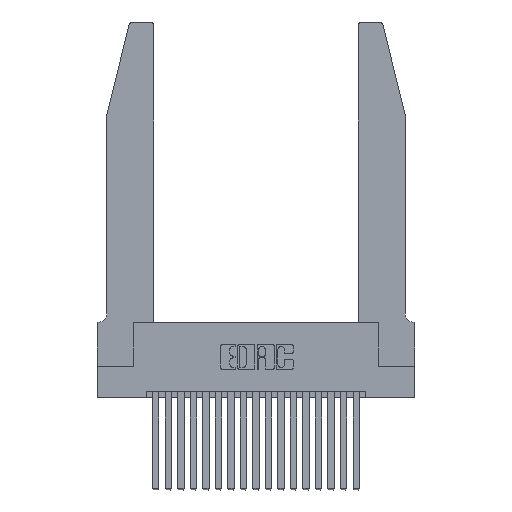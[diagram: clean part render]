
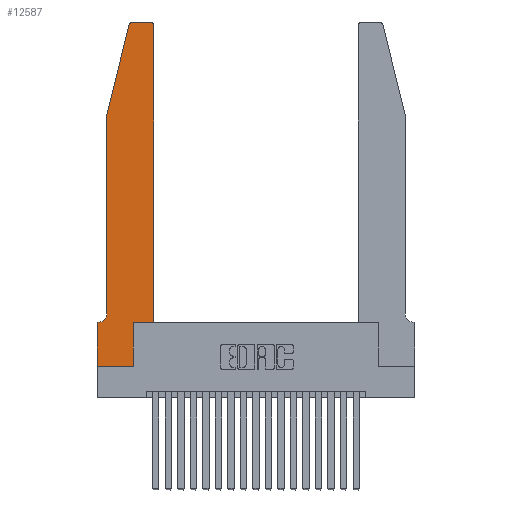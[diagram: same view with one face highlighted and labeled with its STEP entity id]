
A CAD part, top view. The second image highlights one B-rep face of the part: STEP entity #12587.
In plain terms, the highlighted planar face has unit normal (0, 0, 1).
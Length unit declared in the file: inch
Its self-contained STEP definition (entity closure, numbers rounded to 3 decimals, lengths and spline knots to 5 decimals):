
#90 = AXIS2_PLACEMENT_3D ( 'NONE', #17555, #7721, #19156 ) ;
#142 = CIRCLE ( 'NONE', #16223, 0.03 ) ;
#225 = CARTESIAN_POINT ( 'NONE',  ( 0., 0.35, 0.37 ) ) ;
#415 = ORIENTED_EDGE ( 'NONE', *, *, #5488, .T. ) ;
#1071 = EDGE_CURVE ( 'NONE', #3192, #15276, #142, .T. ) ;
#1160 = CARTESIAN_POINT ( 'NONE',  ( 0.4505, 2.72, 0.37 ) ) ;
#1210 = VERTEX_POINT ( 'NONE', #2803 ) ;
#1332 = VERTEX_POINT ( 'NONE', #20515 ) ;
#1396 = VECTOR ( 'NONE', #13830, 39.37008 ) ;
#1727 = EDGE_CURVE ( 'NONE', #9490, #1210, #19424, .T. ) ;
#2191 = CARTESIAN_POINT ( 'NONE',  ( 0.2605, 2.75, 0.37 ) ) ;
#2251 = ORIENTED_EDGE ( 'NONE', *, *, #4260, .T. ) ;
#2430 = DIRECTION ( 'NONE',  ( 0., -1., 0. ) ) ;
#2458 = CARTESIAN_POINT ( 'NONE',  ( 0.284, 2.72, 0.37 ) ) ;
#2617 = CARTESIAN_POINT ( 'NONE',  ( 0.0755, 2., 0.37 ) ) ;
#2803 = CARTESIAN_POINT ( 'NONE',  ( 0.2865, 0., 0.37 ) ) ;
#3170 = VECTOR ( 'NONE', #2430, 39.37008 ) ;
#3192 = VERTEX_POINT ( 'NONE', #1160 ) ;
#3235 = PLANE ( 'NONE',  #4447 ) ;
#3424 = DIRECTION ( 'NONE',  ( 0., 1., 0. ) ) ;
#4129 = DIRECTION ( 'NONE',  ( 1., 0., 0. ) ) ;
#4177 = VECTOR ( 'NONE', #3424, 39.37008 ) ;
#4260 = EDGE_CURVE ( 'NONE', #5948, #15786, #7565, .T. ) ;
#4340 = ORIENTED_EDGE ( 'NONE', *, *, #1727, .T. ) ;
#4447 = AXIS2_PLACEMENT_3D ( 'NONE', #4889, #18024, #8219 ) ;
#4584 = ORIENTED_EDGE ( 'NONE', *, *, #9230, .T. ) ;
#4853 = CIRCLE ( 'NONE', #7307, 0.03 ) ;
#4889 = CARTESIAN_POINT ( 'NONE',  ( 0., 0.35, 0.37 ) ) ;
#5072 = EDGE_CURVE ( 'NONE', #18953, #5948, #6238, .T. ) ;
#5488 = EDGE_CURVE ( 'NONE', #1210, #11672, #20281, .T. ) ;
#5564 = DIRECTION ( 'NONE',  ( 0., 1., 0. ) ) ;
#5693 = CARTESIAN_POINT ( 'NONE',  ( 0.0755, 2., 0.37 ) ) ;
#5948 = VERTEX_POINT ( 'NONE', #11759 ) ;
#5994 = VERTEX_POINT ( 'NONE', #225 ) ;
#6238 = LINE ( 'NONE', #2617, #15561 ) ;
#7248 = CARTESIAN_POINT ( 'NONE',  ( 0.0755, 0.42, 0.37 ) ) ;
#7307 = AXIS2_PLACEMENT_3D ( 'NONE', #2458, #14100, #4129 ) ;
#7374 = EDGE_CURVE ( 'NONE', #15218, #18953, #4853, .T. ) ;
#7511 = DIRECTION ( 'NONE',  ( 1., 0., 0. ) ) ;
#7565 = LINE ( 'NONE', #5693, #3170 ) ;
#7703 = ORIENTED_EDGE ( 'NONE', *, *, #9521, .T. ) ;
#7721 = DIRECTION ( 'NONE',  ( 0., 0., -1. ) ) ;
#8217 = ORIENTED_EDGE ( 'NONE', *, *, #12409, .T. ) ;
#8219 = DIRECTION ( 'NONE',  ( 1., 0., 0. ) ) ;
#8414 = CARTESIAN_POINT ( 'NONE',  ( 0.4205, 2.72, 0.37 ) ) ;
#8636 = DIRECTION ( 'NONE',  ( 0., 0., 1. ) ) ;
#9066 = CARTESIAN_POINT ( 'NONE',  ( 0.0055, 0.35, 0.37 ) ) ;
#9230 = EDGE_CURVE ( 'NONE', #15276, #15218, #14153, .T. ) ;
#9447 = CARTESIAN_POINT ( 'NONE',  ( 0.0755, 0.35, 0.37 ) ) ;
#9490 = VERTEX_POINT ( 'NONE', #11079 ) ;
#9521 = EDGE_CURVE ( 'NONE', #17833, #5994, #18108, .T. ) ;
#9543 = ORIENTED_EDGE ( 'NONE', *, *, #7374, .T. ) ;
#9700 = EDGE_CURVE ( 'NONE', #11672, #1332, #14630, .T. ) ;
#9877 = DIRECTION ( 'NONE',  ( 1., 0., 0. ) ) ;
#10215 = VECTOR ( 'NONE', #9877, 39.37008 ) ;
#10325 = ORIENTED_EDGE ( 'NONE', *, *, #1071, .T. ) ;
#11079 = CARTESIAN_POINT ( 'NONE',  ( 0., 0., 0.37 ) ) ;
#11116 = CARTESIAN_POINT ( 'NONE',  ( 0., 0., 0.37 ) ) ;
#11672 = VERTEX_POINT ( 'NONE', #17099 ) ;
#11759 = CARTESIAN_POINT ( 'NONE',  ( 0.0755, 2., 0.37 ) ) ;
#12409 = EDGE_CURVE ( 'NONE', #5994, #9490, #14084, .T. ) ;
#12540 = DIRECTION ( 'NONE',  ( -0.239, -0.971, 0. ) ) ;
#12587 = ADVANCED_FACE ( 'NONE', ( #19051 ), #3235, .T. ) ;
#12819 = DIRECTION ( 'NONE',  ( -1., 0., 0. ) ) ;
#13212 = EDGE_CURVE ( 'NONE', #1332, #3192, #18293, .T. ) ;
#13617 = CIRCLE ( 'NONE', #90, 0.07 ) ;
#13710 = ORIENTED_EDGE ( 'NONE', *, *, #9700, .T. ) ;
#13830 = DIRECTION ( 'NONE',  ( -1., 0., 0. ) ) ;
#14069 = CARTESIAN_POINT ( 'NONE',  ( 0.4205, 2.75, 0.37 ) ) ;
#14084 = LINE ( 'NONE', #11116, #17814 ) ;
#14100 = DIRECTION ( 'NONE',  ( 0., 0., 1. ) ) ;
#14153 = LINE ( 'NONE', #2191, #1396 ) ;
#14630 = LINE ( 'NONE', #21226, #10215 ) ;
#15015 = CARTESIAN_POINT ( 'NONE',  ( 0.4505, 0.35, 0.37 ) ) ;
#15031 = DIRECTION ( 'NONE',  ( 1., 0., 0. ) ) ;
#15181 = VECTOR ( 'NONE', #15031, 39.37008 ) ;
#15218 = VERTEX_POINT ( 'NONE', #18647 ) ;
#15276 = VERTEX_POINT ( 'NONE', #14069 ) ;
#15481 = CARTESIAN_POINT ( 'NONE',  ( 0.2865, 0.35, 0.37 ) ) ;
#15561 = VECTOR ( 'NONE', #12540, 39.37008 ) ;
#15786 = VERTEX_POINT ( 'NONE', #7248 ) ;
#16044 = VECTOR ( 'NONE', #5564, 39.37008 ) ;
#16223 = AXIS2_PLACEMENT_3D ( 'NONE', #8414, #8636, #7511 ) ;
#17099 = CARTESIAN_POINT ( 'NONE',  ( 0.2865, 0.35, 0.37 ) ) ;
#17403 = CARTESIAN_POINT ( 'NONE',  ( 0.25487, 2.72718, 0.37 ) ) ;
#17555 = CARTESIAN_POINT ( 'NONE',  ( 0.0055, 0.42, 0.37 ) ) ;
#17630 = VECTOR ( 'NONE', #12819, 39.37008 ) ;
#17758 = CARTESIAN_POINT ( 'NONE',  ( 0., 0., 0.37 ) ) ;
#17771 = EDGE_LOOP ( 'NONE', ( #4584, #9543, #18691, #2251, #19698, #7703, #8217, #4340, #415, #13710, #18429, #10325 ) ) ;
#17814 = VECTOR ( 'NONE', #20764, 39.37008 ) ;
#17833 = VERTEX_POINT ( 'NONE', #9066 ) ;
#18024 = DIRECTION ( 'NONE',  ( 0., 0., 1. ) ) ;
#18108 = LINE ( 'NONE', #9447, #17630 ) ;
#18293 = LINE ( 'NONE', #15015, #4177 ) ;
#18429 = ORIENTED_EDGE ( 'NONE', *, *, #13212, .T. ) ;
#18568 = EDGE_CURVE ( 'NONE', #15786, #17833, #13617, .T. ) ;
#18647 = CARTESIAN_POINT ( 'NONE',  ( 0.284, 2.75, 0.37 ) ) ;
#18691 = ORIENTED_EDGE ( 'NONE', *, *, #5072, .T. ) ;
#18953 = VERTEX_POINT ( 'NONE', #17403 ) ;
#19051 = FACE_OUTER_BOUND ( 'NONE', #17771, .T. ) ;
#19156 = DIRECTION ( 'NONE',  ( -1., 0., 0. ) ) ;
#19424 = LINE ( 'NONE', #17758, #15181 ) ;
#19698 = ORIENTED_EDGE ( 'NONE', *, *, #18568, .T. ) ;
#20281 = LINE ( 'NONE', #15481, #16044 ) ;
#20515 = CARTESIAN_POINT ( 'NONE',  ( 0.4505, 0.35, 0.37 ) ) ;
#20764 = DIRECTION ( 'NONE',  ( 0., -1., 0. ) ) ;
#21226 = CARTESIAN_POINT ( 'NONE',  ( 0.4505, 0.35, 0.37 ) ) ;
